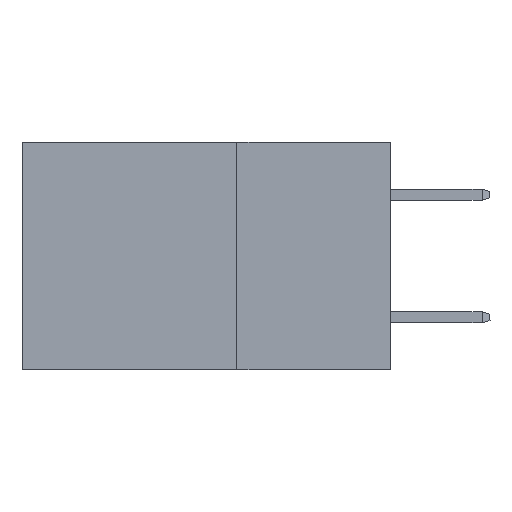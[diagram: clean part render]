
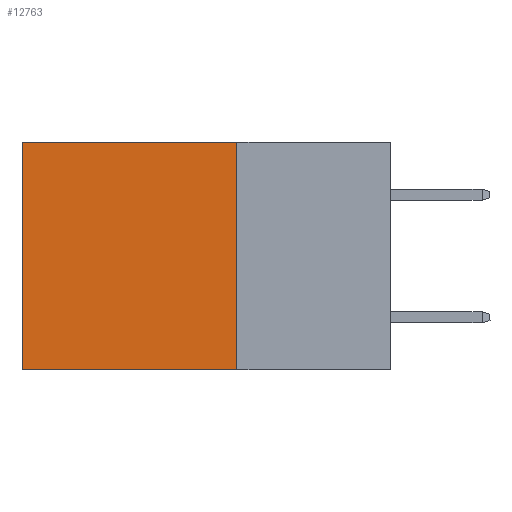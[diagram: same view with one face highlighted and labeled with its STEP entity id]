
A CAD part, left-side view. The second image highlights one B-rep face of the part: STEP entity #12763.
In plain terms, the highlighted planar face has unit normal (-1, 0, 0).
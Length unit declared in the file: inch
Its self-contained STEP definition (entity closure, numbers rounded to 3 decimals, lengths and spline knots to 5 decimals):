
#933 = DIRECTION ( 'NONE',  ( 0., 0., -1. ) ) ;
#980 = EDGE_LOOP ( 'NONE', ( #15367, #14086, #11303, #7391 ) ) ;
#1597 = VECTOR ( 'NONE', #10321, 39.37008 ) ;
#1746 = VECTOR ( 'NONE', #933, 39.37008 ) ;
#1761 = LINE ( 'NONE', #6670, #1597 ) ;
#2041 = AXIS2_PLACEMENT_3D ( 'NONE', #14219, #10346, #14138 ) ;
#2198 = DIRECTION ( 'NONE',  ( 0., 0., -1. ) ) ;
#2269 = CARTESIAN_POINT ( 'NONE',  ( 0.2875, 0.25, 0. ) ) ;
#2367 = EDGE_CURVE ( 'NONE', #9430, #5519, #3317, .T. ) ;
#2817 = CARTESIAN_POINT ( 'NONE',  ( 0.2875, 0.6, -0.37 ) ) ;
#3317 = LINE ( 'NONE', #2269, #12444 ) ;
#5344 = EDGE_CURVE ( 'NONE', #14856, #14349, #6723, .T. ) ;
#5519 = VERTEX_POINT ( 'NONE', #15906 ) ;
#6670 = CARTESIAN_POINT ( 'NONE',  ( 0.2875, 0.25, -0.37 ) ) ;
#6723 = LINE ( 'NONE', #7035, #1746 ) ;
#7035 = CARTESIAN_POINT ( 'NONE',  ( 0.2875, 0.6, 0. ) ) ;
#7391 = ORIENTED_EDGE ( 'NONE', *, *, #7919, .T. ) ;
#7919 = EDGE_CURVE ( 'NONE', #9430, #14856, #13293, .T. ) ;
#9079 = EDGE_CURVE ( 'NONE', #5519, #14349, #1761, .T. ) ;
#9430 = VERTEX_POINT ( 'NONE', #12634 ) ;
#9564 = CARTESIAN_POINT ( 'NONE',  ( 0.2875, 0.25, 0. ) ) ;
#10321 = DIRECTION ( 'NONE',  ( 0., 1., 0. ) ) ;
#10346 = DIRECTION ( 'NONE',  ( 1., 0., 0. ) ) ;
#10776 = DIRECTION ( 'NONE',  ( 0., 1., 0. ) ) ;
#11303 = ORIENTED_EDGE ( 'NONE', *, *, #2367, .F. ) ;
#11316 = CARTESIAN_POINT ( 'NONE',  ( 0.2875, 0.6, 0. ) ) ;
#11550 = FACE_OUTER_BOUND ( 'NONE', #980, .T. ) ;
#12395 = VECTOR ( 'NONE', #10776, 39.37008 ) ;
#12444 = VECTOR ( 'NONE', #2198, 39.37008 ) ;
#12634 = CARTESIAN_POINT ( 'NONE',  ( 0.2875, 0.25, 0. ) ) ;
#12763 = ADVANCED_FACE ( 'NONE', ( #11550 ), #13078, .F. ) ;
#13078 = PLANE ( 'NONE',  #2041 ) ;
#13293 = LINE ( 'NONE', #9564, #12395 ) ;
#14086 = ORIENTED_EDGE ( 'NONE', *, *, #9079, .F. ) ;
#14138 = DIRECTION ( 'NONE',  ( 0., 0., -1. ) ) ;
#14219 = CARTESIAN_POINT ( 'NONE',  ( 0.2875, 0.25, 0. ) ) ;
#14349 = VERTEX_POINT ( 'NONE', #2817 ) ;
#14856 = VERTEX_POINT ( 'NONE', #11316 ) ;
#15367 = ORIENTED_EDGE ( 'NONE', *, *, #5344, .T. ) ;
#15906 = CARTESIAN_POINT ( 'NONE',  ( 0.2875, 0.25, -0.37 ) ) ;
